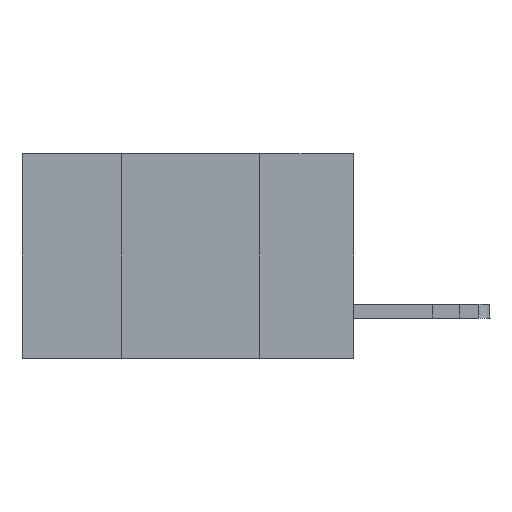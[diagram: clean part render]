
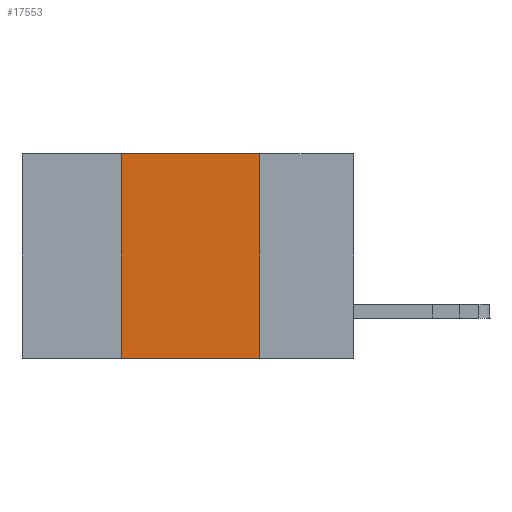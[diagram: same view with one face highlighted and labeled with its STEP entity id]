
A CAD part, left-side view. The second image highlights one B-rep face of the part: STEP entity #17553.
In plain terms, the highlighted planar face has unit normal (-1, 0, 0).
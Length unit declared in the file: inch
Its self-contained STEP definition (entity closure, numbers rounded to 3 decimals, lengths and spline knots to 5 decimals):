
#1258 = PLANE ( 'NONE',  #20493 ) ;
#1733 = CARTESIAN_POINT ( 'NONE',  ( 0., 0.17, 0. ) ) ;
#2056 = DIRECTION ( 'NONE',  ( 0., 0., -1. ) ) ;
#3198 = ORIENTED_EDGE ( 'NONE', *, *, #16998, .T. ) ;
#5902 = CARTESIAN_POINT ( 'NONE',  ( 0., 0.17, -0.37 ) ) ;
#7363 = DIRECTION ( 'NONE',  ( 0., -1., 0. ) ) ;
#8171 = EDGE_CURVE ( 'NONE', #29980, #12331, #25304, .T. ) ;
#8644 = CARTESIAN_POINT ( 'NONE',  ( 0., 0.17, 0. ) ) ;
#9098 = VECTOR ( 'NONE', #7363, 39.37008 ) ;
#9473 = VECTOR ( 'NONE', #17038, 39.37008 ) ;
#10049 = CARTESIAN_POINT ( 'NONE',  ( 0., 0.6, -0.37 ) ) ;
#11312 = DIRECTION ( 'NONE',  ( 0., 0., -1. ) ) ;
#11498 = ORIENTED_EDGE ( 'NONE', *, *, #8171, .F. ) ;
#12099 = VECTOR ( 'NONE', #25662, 39.37008 ) ;
#12331 = VERTEX_POINT ( 'NONE', #8644 ) ;
#13631 = CARTESIAN_POINT ( 'NONE',  ( 0., 0.42, -0.37 ) ) ;
#14780 = VERTEX_POINT ( 'NONE', #13631 ) ;
#16998 = EDGE_CURVE ( 'NONE', #14780, #29111, #30858, .T. ) ;
#17038 = DIRECTION ( 'NONE',  ( 0., -1., 0. ) ) ;
#17553 = ADVANCED_FACE ( 'NONE', ( #21637 ), #1258, .F. ) ;
#19007 = EDGE_LOOP ( 'NONE', ( #24779, #11498, #20939, #3198 ) ) ;
#20493 = AXIS2_PLACEMENT_3D ( 'NONE', #26142, #31178, #11312 ) ;
#20939 = ORIENTED_EDGE ( 'NONE', *, *, #29156, .F. ) ;
#21637 = FACE_OUTER_BOUND ( 'NONE', #19007, .T. ) ;
#22118 = LINE ( 'NONE', #1733, #31071 ) ;
#24083 = CARTESIAN_POINT ( 'NONE',  ( 0., 0.42, 0. ) ) ;
#24779 = ORIENTED_EDGE ( 'NONE', *, *, #25156, .F. ) ;
#25156 = EDGE_CURVE ( 'NONE', #12331, #29111, #22118, .T. ) ;
#25304 = LINE ( 'NONE', #30415, #9473 ) ;
#25662 = DIRECTION ( 'NONE',  ( 0., 0., 1. ) ) ;
#26142 = CARTESIAN_POINT ( 'NONE',  ( 0., 0.6, 0. ) ) ;
#27653 = LINE ( 'NONE', #30341, #12099 ) ;
#29111 = VERTEX_POINT ( 'NONE', #5902 ) ;
#29156 = EDGE_CURVE ( 'NONE', #14780, #29980, #27653, .T. ) ;
#29980 = VERTEX_POINT ( 'NONE', #24083 ) ;
#30341 = CARTESIAN_POINT ( 'NONE',  ( 0., 0.42, 0. ) ) ;
#30415 = CARTESIAN_POINT ( 'NONE',  ( 0., 0.6, 0. ) ) ;
#30858 = LINE ( 'NONE', #10049, #9098 ) ;
#31071 = VECTOR ( 'NONE', #2056, 39.37008 ) ;
#31178 = DIRECTION ( 'NONE',  ( 1., 0., 0. ) ) ;
